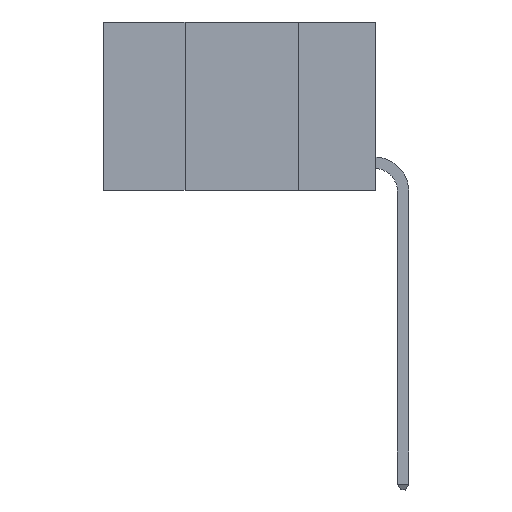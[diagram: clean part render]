
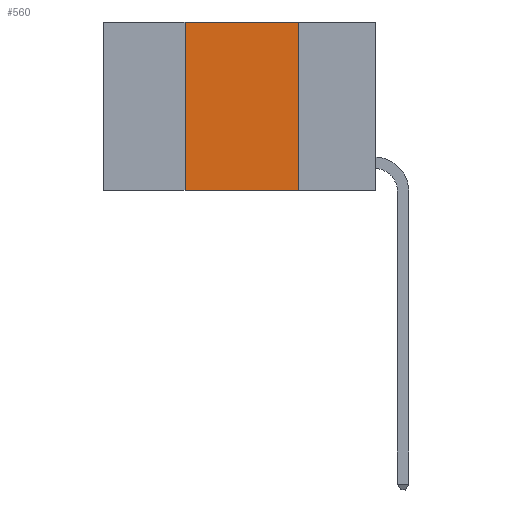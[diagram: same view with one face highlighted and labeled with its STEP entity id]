
A CAD part, left-side view. The second image highlights one B-rep face of the part: STEP entity #560.
In plain terms, the highlighted planar face has unit normal (-1, 0, 0).
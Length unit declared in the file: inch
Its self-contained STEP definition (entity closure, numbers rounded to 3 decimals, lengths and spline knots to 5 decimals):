
#43 = CARTESIAN_POINT ( 'NONE',  ( 0., 0.42, 0. ) ) ;
#449 = DIRECTION ( 'NONE',  ( 0., 0., -1. ) ) ;
#560 = ADVANCED_FACE ( 'NONE', ( #5599 ), #2950, .F. ) ;
#775 = CARTESIAN_POINT ( 'NONE',  ( 0., 0.17, -0.37 ) ) ;
#1049 = CARTESIAN_POINT ( 'NONE',  ( 0., 0.17, 0. ) ) ;
#1118 = ORIENTED_EDGE ( 'NONE', *, *, #4353, .F. ) ;
#1237 = DIRECTION ( 'NONE',  ( 0., 0., 1. ) ) ;
#1382 = ORIENTED_EDGE ( 'NONE', *, *, #8940, .T. ) ;
#2260 = DIRECTION ( 'NONE',  ( 0., -1., 0. ) ) ;
#2271 = CARTESIAN_POINT ( 'NONE',  ( 0., 0.42, -0.37 ) ) ;
#2925 = VECTOR ( 'NONE', #1237, 39.37008 ) ;
#2950 = PLANE ( 'NONE',  #10440 ) ;
#3042 = ORIENTED_EDGE ( 'NONE', *, *, #10133, .F. ) ;
#3707 = CARTESIAN_POINT ( 'NONE',  ( 0., 0.42, 0. ) ) ;
#4127 = VECTOR ( 'NONE', #5922, 39.37008 ) ;
#4353 = EDGE_CURVE ( 'NONE', #7862, #8356, #9067, .T. ) ;
#4594 = CARTESIAN_POINT ( 'NONE',  ( 0., 0.6, 0. ) ) ;
#5385 = DIRECTION ( 'NONE',  ( 1., 0., 0. ) ) ;
#5599 = FACE_OUTER_BOUND ( 'NONE', #5701, .T. ) ;
#5695 = VERTEX_POINT ( 'NONE', #775 ) ;
#5701 = EDGE_LOOP ( 'NONE', ( #9529, #1118, #3042, #1382 ) ) ;
#5922 = DIRECTION ( 'NONE',  ( 0., -1., 0. ) ) ;
#6217 = LINE ( 'NONE', #7517, #4127 ) ;
#6261 = CARTESIAN_POINT ( 'NONE',  ( 0., 0.6, 0. ) ) ;
#6718 = VECTOR ( 'NONE', #2260, 39.37008 ) ;
#6997 = VERTEX_POINT ( 'NONE', #2271 ) ;
#7239 = LINE ( 'NONE', #3707, #2925 ) ;
#7274 = CARTESIAN_POINT ( 'NONE',  ( 0., 0.17, 0. ) ) ;
#7517 = CARTESIAN_POINT ( 'NONE',  ( 0., 0.6, -0.37 ) ) ;
#7568 = DIRECTION ( 'NONE',  ( 0., 0., -1. ) ) ;
#7862 = VERTEX_POINT ( 'NONE', #43 ) ;
#7962 = EDGE_CURVE ( 'NONE', #8356, #5695, #9820, .T. ) ;
#8356 = VERTEX_POINT ( 'NONE', #7274 ) ;
#8940 = EDGE_CURVE ( 'NONE', #6997, #5695, #6217, .T. ) ;
#9067 = LINE ( 'NONE', #6261, #6718 ) ;
#9529 = ORIENTED_EDGE ( 'NONE', *, *, #7962, .F. ) ;
#9820 = LINE ( 'NONE', #1049, #10050 ) ;
#10050 = VECTOR ( 'NONE', #7568, 39.37008 ) ;
#10133 = EDGE_CURVE ( 'NONE', #6997, #7862, #7239, .T. ) ;
#10440 = AXIS2_PLACEMENT_3D ( 'NONE', #4594, #5385, #449 ) ;
